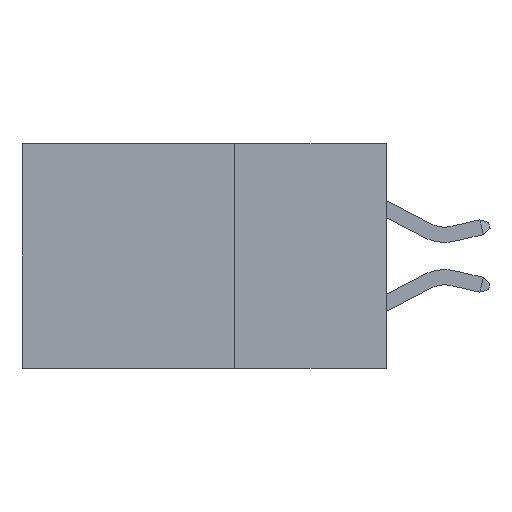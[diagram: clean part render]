
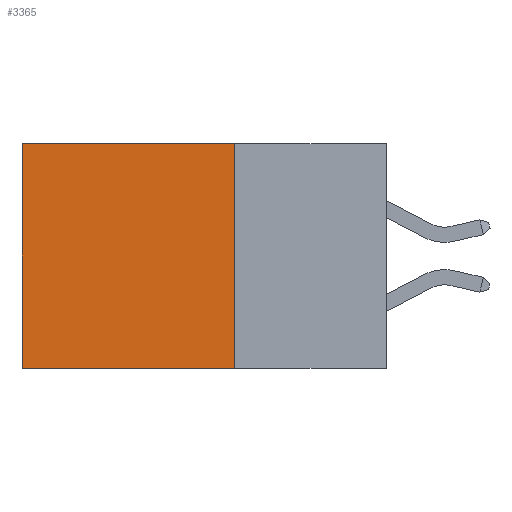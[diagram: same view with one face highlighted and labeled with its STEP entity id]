
A CAD part, left-side view. The second image highlights one B-rep face of the part: STEP entity #3365.
In plain terms, the highlighted planar face has unit normal (-1, 0, 0).
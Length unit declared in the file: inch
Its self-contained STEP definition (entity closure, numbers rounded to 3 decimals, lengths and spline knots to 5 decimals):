
#178 = EDGE_CURVE ( 'NONE', #9585, #6958, #1955, .T. ) ;
#368 = ORIENTED_EDGE ( 'NONE', *, *, #6620, .T. ) ;
#392 = EDGE_CURVE ( 'NONE', #9632, #6958, #1794, .T. ) ;
#1180 = LINE ( 'NONE', #1925, #5594 ) ;
#1794 = LINE ( 'NONE', #5777, #6078 ) ;
#1925 = CARTESIAN_POINT ( 'NONE',  ( 0.298, 0.25, 0. ) ) ;
#1955 = LINE ( 'NONE', #7870, #4697 ) ;
#2852 = EDGE_CURVE ( 'NONE', #6441, #9585, #1180, .T. ) ;
#3365 = ADVANCED_FACE ( 'NONE', ( #7647 ), #3993, .F. ) ;
#3838 = AXIS2_PLACEMENT_3D ( 'NONE', #4037, #5255, #5276 ) ;
#3993 = PLANE ( 'NONE',  #3838 ) ;
#4037 = CARTESIAN_POINT ( 'NONE',  ( 0.298, 0.25, 0. ) ) ;
#4391 = ORIENTED_EDGE ( 'NONE', *, *, #178, .F. ) ;
#4449 = ORIENTED_EDGE ( 'NONE', *, *, #2852, .F. ) ;
#4697 = VECTOR ( 'NONE', #9262, 39.37008 ) ;
#4784 = CARTESIAN_POINT ( 'NONE',  ( 0.298, 0.6, 0. ) ) ;
#5255 = DIRECTION ( 'NONE',  ( 1., 0., 0. ) ) ;
#5276 = DIRECTION ( 'NONE',  ( 0., 0., -1. ) ) ;
#5542 = VECTOR ( 'NONE', #6215, 39.37008 ) ;
#5594 = VECTOR ( 'NONE', #7274, 39.37008 ) ;
#5777 = CARTESIAN_POINT ( 'NONE',  ( 0.298, 0.6, 0. ) ) ;
#5881 = CARTESIAN_POINT ( 'NONE',  ( 0.298, 0.6, -0.37 ) ) ;
#6078 = VECTOR ( 'NONE', #8214, 39.37008 ) ;
#6215 = DIRECTION ( 'NONE',  ( 0., 1., 0. ) ) ;
#6441 = VERTEX_POINT ( 'NONE', #10396 ) ;
#6620 = EDGE_CURVE ( 'NONE', #6441, #9632, #7341, .T. ) ;
#6958 = VERTEX_POINT ( 'NONE', #5881 ) ;
#7274 = DIRECTION ( 'NONE',  ( 0., 0., -1. ) ) ;
#7299 = EDGE_LOOP ( 'NONE', ( #9580, #4391, #4449, #368 ) ) ;
#7341 = LINE ( 'NONE', #10690, #5542 ) ;
#7647 = FACE_OUTER_BOUND ( 'NONE', #7299, .T. ) ;
#7870 = CARTESIAN_POINT ( 'NONE',  ( 0.298, 0.25, -0.37 ) ) ;
#7907 = CARTESIAN_POINT ( 'NONE',  ( 0.298, 0.25, -0.37 ) ) ;
#8214 = DIRECTION ( 'NONE',  ( 0., 0., -1. ) ) ;
#9262 = DIRECTION ( 'NONE',  ( 0., 1., 0. ) ) ;
#9580 = ORIENTED_EDGE ( 'NONE', *, *, #392, .T. ) ;
#9585 = VERTEX_POINT ( 'NONE', #7907 ) ;
#9632 = VERTEX_POINT ( 'NONE', #4784 ) ;
#10396 = CARTESIAN_POINT ( 'NONE',  ( 0.298, 0.25, 0. ) ) ;
#10690 = CARTESIAN_POINT ( 'NONE',  ( 0.298, 0.25, 0. ) ) ;
